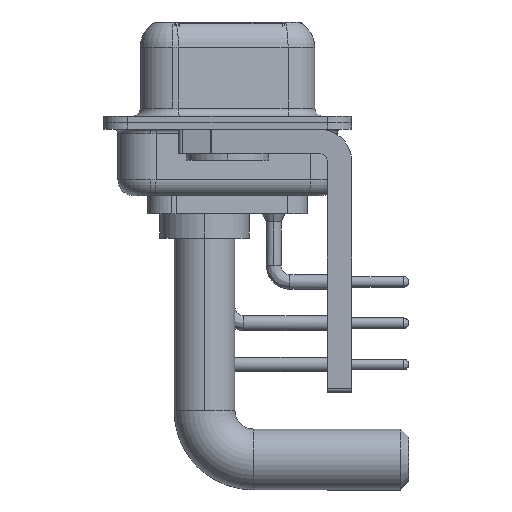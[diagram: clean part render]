
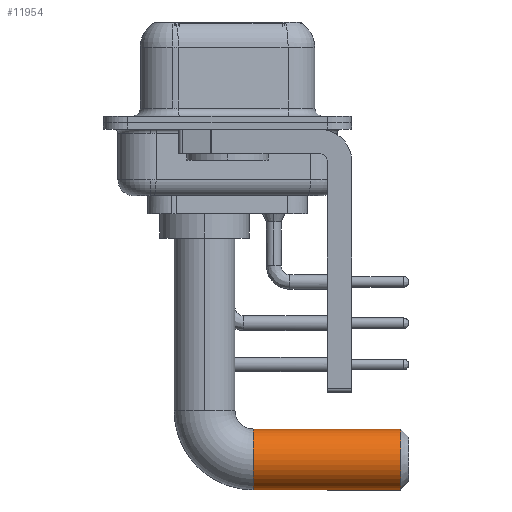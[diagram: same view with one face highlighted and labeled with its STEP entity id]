
A CAD part, left-side view. The second image highlights one B-rep face of the part: STEP entity #11954.
In plain terms, the highlighted cylindrical face has radius 1.875 mm (diameter 3.75 mm), a partial arc.
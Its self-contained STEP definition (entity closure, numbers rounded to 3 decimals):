
#464 = VERTEX_POINT ( 'NONE', #28586 ) ;
#493 = CARTESIAN_POINT ( 'NONE',  ( 0., -3., -13.63 ) ) ;
#1341 = ORIENTED_EDGE ( 'NONE', *, *, #21549, .T. ) ;
#1370 = CIRCLE ( 'NONE', #25208, 1.875 ) ;
#1385 = CARTESIAN_POINT ( 'NONE',  ( 0., -12.07, -13.63 ) ) ;
#1663 = LINE ( 'NONE', #20560, #12587 ) ;
#1824 = CIRCLE ( 'NONE', #27099, 1.875 ) ;
#3665 = DIRECTION ( 'NONE',  ( 0., 0., -1. ) ) ;
#4282 = DIRECTION ( 'NONE',  ( 0., -1., 0. ) ) ;
#5739 = EDGE_LOOP ( 'NONE', ( #6324, #11077, #1341, #20963 ) ) ;
#6324 = ORIENTED_EDGE ( 'NONE', *, *, #22399, .F. ) ;
#6448 = VERTEX_POINT ( 'NONE', #11557 ) ;
#6897 = DIRECTION ( 'NONE',  ( 0., -1., 0. ) ) ;
#8837 = VERTEX_POINT ( 'NONE', #24521 ) ;
#8840 = FACE_OUTER_BOUND ( 'NONE', #5739, .T. ) ;
#10535 = DIRECTION ( 'NONE',  ( 0., 1., 0. ) ) ;
#10968 = DIRECTION ( 'NONE',  ( 0., -1., 0. ) ) ;
#11077 = ORIENTED_EDGE ( 'NONE', *, *, #21602, .T. ) ;
#11557 = CARTESIAN_POINT ( 'NONE',  ( 0., -3., -11.755 ) ) ;
#11954 = ADVANCED_FACE ( 'NONE', ( #8840 ), #18145, .T. ) ;
#12526 = DIRECTION ( 'NONE',  ( 0., -1., 0. ) ) ;
#12587 = VECTOR ( 'NONE', #10968, 1000. ) ;
#13572 = DIRECTION ( 'NONE',  ( 0., 0., -1. ) ) ;
#15259 = VERTEX_POINT ( 'NONE', #25990 ) ;
#15481 = VECTOR ( 'NONE', #6897, 1000. ) ;
#18145 = CYLINDRICAL_SURFACE ( 'NONE', #20433, 1.875 ) ;
#20433 = AXIS2_PLACEMENT_3D ( 'NONE', #25133, #4282, #13572 ) ;
#20560 = CARTESIAN_POINT ( 'NONE',  ( 0., -3., -11.755 ) ) ;
#20772 = LINE ( 'NONE', #27755, #15481 ) ;
#20963 = ORIENTED_EDGE ( 'NONE', *, *, #21793, .T. ) ;
#21519 = DIRECTION ( 'NONE',  ( -1., 0., 0. ) ) ;
#21549 = EDGE_CURVE ( 'NONE', #8837, #15259, #20772, .T. ) ;
#21602 = EDGE_CURVE ( 'NONE', #6448, #8837, #1824, .T. ) ;
#21793 = EDGE_CURVE ( 'NONE', #15259, #464, #1370, .T. ) ;
#22399 = EDGE_CURVE ( 'NONE', #6448, #464, #1663, .T. ) ;
#24521 = CARTESIAN_POINT ( 'NONE',  ( 0., -3., -15.505 ) ) ;
#25133 = CARTESIAN_POINT ( 'NONE',  ( 0., -3., -13.63 ) ) ;
#25208 = AXIS2_PLACEMENT_3D ( 'NONE', #1385, #10535, #3665 ) ;
#25990 = CARTESIAN_POINT ( 'NONE',  ( 0., -12.07, -15.505 ) ) ;
#27099 = AXIS2_PLACEMENT_3D ( 'NONE', #493, #12526, #21519 ) ;
#27755 = CARTESIAN_POINT ( 'NONE',  ( 0., -3., -15.505 ) ) ;
#28586 = CARTESIAN_POINT ( 'NONE',  ( 0., -12.07, -11.755 ) ) ;
